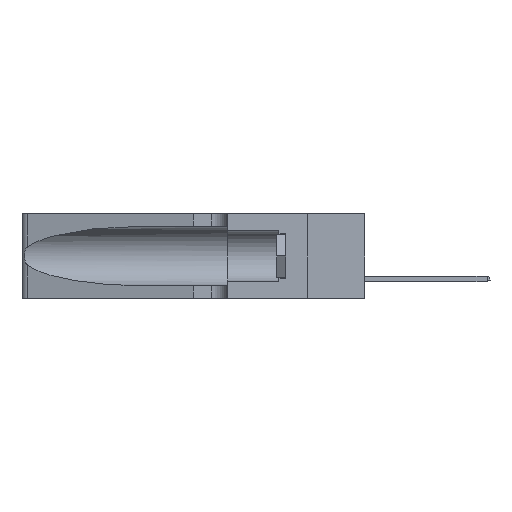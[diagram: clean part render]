
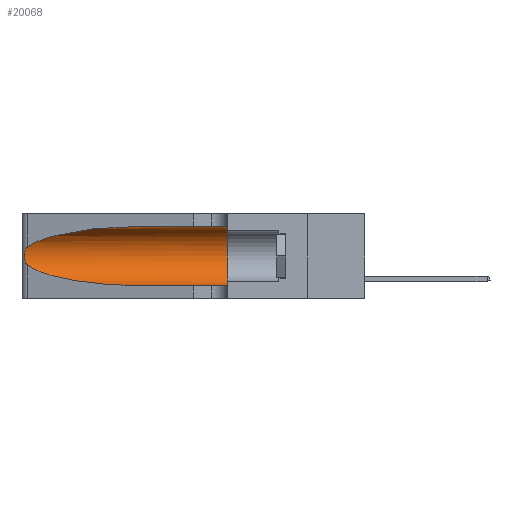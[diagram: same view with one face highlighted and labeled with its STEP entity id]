
A CAD part, left-side view. The second image highlights one B-rep face of the part: STEP entity #20068.
In plain terms, the highlighted cylindrical face has radius 3.308 mm (diameter 6.617 mm), a partial arc.
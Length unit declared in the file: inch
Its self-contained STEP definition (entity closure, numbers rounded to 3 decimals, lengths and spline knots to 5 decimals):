
#737 = DIRECTION ( 'NONE',  ( 0., -1., 0. ) ) ;
#1166 = AXIS2_PLACEMENT_3D ( 'NONE', #2784, #27770, #6841 ) ;
#1878 = CARTESIAN_POINT ( 'NONE',  ( 0.1305, 1.61858, 0.31525 ) ) ;
#2017 = CARTESIAN_POINT ( 'NONE',  ( 0.25555, 1.22993, 0.14849 ) ) ;
#2784 = CARTESIAN_POINT ( 'NONE',  ( 0.1305, 0.35, 0.185 ) ) ;
#4260 = CARTESIAN_POINT ( 'NONE',  ( 0.2373, 1.15595, 0.08982 ) ) ;
#5038 = CARTESIAN_POINT ( 'NONE',  ( 0.25639, 1.23184, 0.21858 ) ) ;
#5196 = CARTESIAN_POINT ( 'NONE',  ( 0.25555, 1.22994, 0.2215 ) ) ;
#5555 = ORIENTED_EDGE ( 'NONE', *, *, #27544, .T. ) ;
#6446 = CARTESIAN_POINT ( 'NONE',  ( 0.25787, 1.23484, 0.2124 ) ) ;
#6733 = VERTEX_POINT ( 'NONE', #35154 ) ;
#6841 = DIRECTION ( 'NONE',  ( 0., 0., 1. ) ) ;
#7642 = VECTOR ( 'NONE', #41232, 39.37008 ) ;
#9083 = ORIENTED_EDGE ( 'NONE', *, *, #21494, .F. ) ;
#10240 = VERTEX_POINT ( 'NONE', #24418 ) ;
#12451 = VERTEX_POINT ( 'NONE', #17161 ) ;
#14028 = AXIS2_PLACEMENT_3D ( 'NONE', #32286, #737, #29042 ) ;
#14584 = VERTEX_POINT ( 'NONE', #26186 ) ;
#14613 = CARTESIAN_POINT ( 'NONE',  ( 0.18966, 0.96281, 0.05475 ) ) ;
#15608 = B_SPLINE_CURVE_WITH_KNOTS ( 'NONE', 3,
 ( #43888, #5196, #5038, #6446, #28017, #25287, #29953, #19642, #22904, #37594, #35555, #43830, #2017, #31041 ),
 .UNSPECIFIED., .F., .F.,
 ( 4, 2, 2, 2, 2, 2, 4 ),
 ( 0., 0.00027, 0.00053, 0.00107, 0.0016, 0.00187, 0.00214 ),
 .UNSPECIFIED. ) ;
#15635 = VERTEX_POINT ( 'NONE', #30627 ) ;
#17161 = CARTESIAN_POINT ( 'NONE',  ( 0.1305, 0.35, 0.31525 ) ) ;
#18537 = CARTESIAN_POINT ( 'NONE',  ( 0.25487, 1.22718, 0.22369 ) ) ;
#19588 = ORIENTED_EDGE ( 'NONE', *, *, #43281, .T. ) ;
#19642 = CARTESIAN_POINT ( 'NONE',  ( 0.26075, 1.23896, 0.178 ) ) ;
#20068 = ADVANCED_FACE ( 'NONE', ( #44088 ), #23423, .F. ) ;
#21170 = EDGE_CURVE ( 'NONE', #35762, #10240, #15608, .T. ) ;
#21494 = EDGE_CURVE ( 'NONE', #15635, #12451, #46169, .T. ) ;
#21883 = EDGE_CURVE ( 'NONE', #12451, #6733, #38377, .T. ) ;
#22031 = CARTESIAN_POINT ( 'NONE',  ( 0.1305, 0.72297, 0.05475 ) ) ;
#22904 = CARTESIAN_POINT ( 'NONE',  ( 0.26017, 1.23833, 0.17102 ) ) ;
#23423 = CYLINDRICAL_SURFACE ( 'NONE', #14028, 0.13025 ) ;
#23473 = CARTESIAN_POINT ( 'NONE',  ( 0.25487, 1.22718, 0.22369 ) ) ;
#24418 = CARTESIAN_POINT ( 'NONE',  ( 0.25487, 1.22718, 0.14631 ) ) ;
#24895 = DIRECTION ( 'NONE',  ( 0., -1., 0. ) ) ;
#25287 = CARTESIAN_POINT ( 'NONE',  ( 0.26018, 1.23835, 0.19895 ) ) ;
#26186 = CARTESIAN_POINT ( 'NONE',  ( 0.1305, 0.72297, 0.05475 ) ) ;
#26478 = CARTESIAN_POINT ( 'NONE',  ( 0.1305, 1.61858, 0.05475 ) ) ;
#27544 = EDGE_CURVE ( 'NONE', #14584, #6733, #32611, .T. ) ;
#27692 = CARTESIAN_POINT ( 'NONE',  ( 0.1305, 0.72297, 0.31525 ) ) ;
#27770 = DIRECTION ( 'NONE',  ( 0., 1., 0. ) ) ;
#28017 = CARTESIAN_POINT ( 'NONE',  ( 0.25854, 1.2359, 0.20912 ) ) ;
#29042 = DIRECTION ( 'NONE',  ( 0., 0., -1. ) ) ;
#29953 = CARTESIAN_POINT ( 'NONE',  ( 0.26075, 1.23896, 0.19203 ) ) ;
#30627 = CARTESIAN_POINT ( 'NONE',  ( 0.1305, 0.72297, 0.31525 ) ) ;
#31041 = CARTESIAN_POINT ( 'NONE',  ( 0.25487, 1.22718, 0.14631 ) ) ;
#31478 = ORIENTED_EDGE ( 'NONE', *, *, #36303, .T. ) ;
#32286 = CARTESIAN_POINT ( 'NONE',  ( 0.1305, 1.61858, 0.185 ) ) ;
#32353 = CARTESIAN_POINT ( 'NONE',  ( 0.25487, 1.22718, 0.14631 ) ) ;
#32601 = CARTESIAN_POINT ( 'NONE',  ( 0.2373, 1.15595, 0.28018 ) ) ;
#32611 = LINE ( 'NONE', #26478, #43768 ) ;
#33740 = ORIENTED_EDGE ( 'NONE', *, *, #21170, .T. ) ;
#35154 = CARTESIAN_POINT ( 'NONE',  ( 0.1305, 0.35, 0.05475 ) ) ;
#35555 = CARTESIAN_POINT ( 'NONE',  ( 0.25789, 1.23486, 0.15765 ) ) ;
#35762 = VERTEX_POINT ( 'NONE', #23473 ) ;
#36287 = EDGE_LOOP ( 'NONE', ( #19588, #33740, #31478, #5555, #36339, #9083 ) ) ;
#36303 = EDGE_CURVE ( 'NONE', #10240, #14584, #44496, .T. ) ;
#36339 = ORIENTED_EDGE ( 'NONE', *, *, #21883, .F. ) ;
#37594 = CARTESIAN_POINT ( 'NONE',  ( 0.25856, 1.23593, 0.16098 ) ) ;
#38252 =( BOUNDED_CURVE ( )  B_SPLINE_CURVE ( 3, ( #27692, #38470, #32601, #18537 ),
 .UNSPECIFIED., .F., .T. ) 
 B_SPLINE_CURVE_WITH_KNOTS ( ( 4, 4 ),
 ( 1.5708, 2.84003 ),
 .UNSPECIFIED. ) 
 CURVE ( )  GEOMETRIC_REPRESENTATION_ITEM ( )  RATIONAL_B_SPLINE_CURVE ( ( 1., 0.87, 0.87, 1. ) ) 
 REPRESENTATION_ITEM ( '' )  );
#38377 = CIRCLE ( 'NONE', #1166, 0.13025 ) ;
#38470 = CARTESIAN_POINT ( 'NONE',  ( 0.18966, 0.96281, 0.31525 ) ) ;
#41232 = DIRECTION ( 'NONE',  ( 0., -1., 0. ) ) ;
#43281 = EDGE_CURVE ( 'NONE', #15635, #35762, #38252, .T. ) ;
#43768 = VECTOR ( 'NONE', #24895, 39.37008 ) ;
#43830 = CARTESIAN_POINT ( 'NONE',  ( 0.25639, 1.23186, 0.15144 ) ) ;
#43888 = CARTESIAN_POINT ( 'NONE',  ( 0.25487, 1.22718, 0.22369 ) ) ;
#44088 = FACE_OUTER_BOUND ( 'NONE', #36287, .T. ) ;
#44496 =( BOUNDED_CURVE ( )  B_SPLINE_CURVE ( 3, ( #32353, #4260, #14613, #22031 ),
 .UNSPECIFIED., .F., .F. ) 
 B_SPLINE_CURVE_WITH_KNOTS ( ( 4, 4 ),
 ( 3.44316, 4.71239 ),
 .UNSPECIFIED. ) 
 CURVE ( )  GEOMETRIC_REPRESENTATION_ITEM ( )  RATIONAL_B_SPLINE_CURVE ( ( 1., 0.87, 0.87, 1. ) ) 
 REPRESENTATION_ITEM ( '' )  );
#46169 = LINE ( 'NONE', #1878, #7642 ) ;
